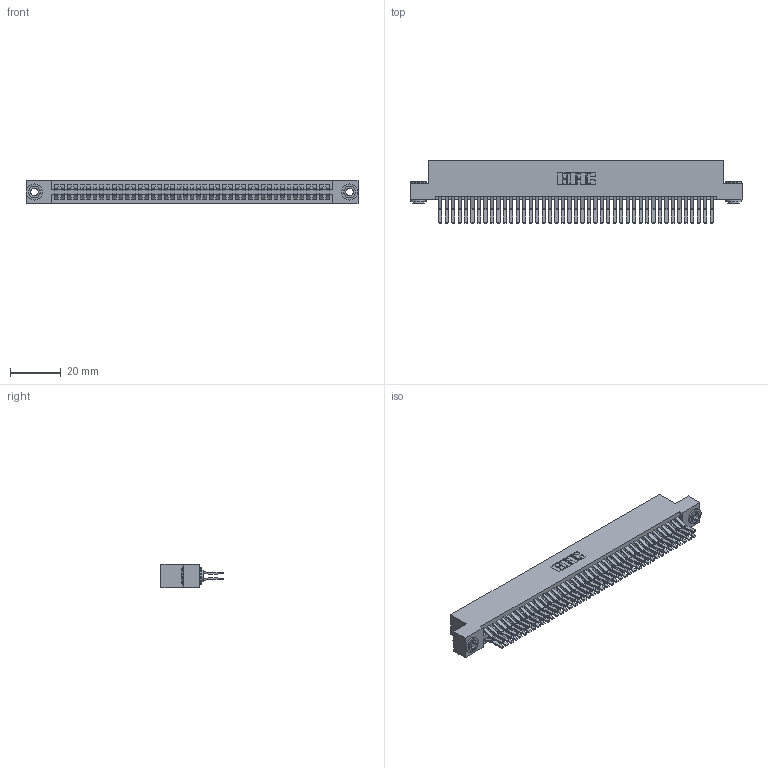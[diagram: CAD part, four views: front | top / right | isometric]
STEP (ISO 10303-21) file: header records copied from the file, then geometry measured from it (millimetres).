
FILE_DESCRIPTION (( 'STEP AP203' ), '1' );
FILE_NAME ('345-086-560-203.STEP', '2019-11-01T09:35:39', ( '' ), ( '' ), 'SwSTEP 2.0', 'SolidWorks 2016', '' );
FILE_SCHEMA (( 'CONFIG_CONTROL_DESIGN' ));
Length unit declared in the file: inch
Products named in the file (4): 345 Part_Flush Mounting Lugs - 0.156 Dia-TH; 345-292-001_560 Tail; 345-086-560-203; 345-250-002_345-250-002-102
Assembly tree (89 placements, depth 2):
  345-086-560-203
    345 Part_Flush Mounting Lugs - 0.156 Dia-TH
    345-292-001_560 Tail  x86
    345-250-002_345-250-002-102  x2
Bounding box: 130.43 x 24.45 x 9.4 mm (x, y, z)
Volume: 13262.4 mm3; surface area: 21278.1 mm2
Topology: 89 solids, 89 shells, 4636 faces, 13747 edges, 9046 vertices
Faces by surface type: plane 2928, cylinder 1700, cone 8
Entity records: 34342 total; most frequent: CARTESIAN_POINT 5731, ORIENTED_EDGE 5658, DIRECTION 5087, EDGE_CURVE 2829, VECTOR 2497, LINE 2497, VERTEX_POINT 1882, AXIS2_PLACEMENT_3D 1295
